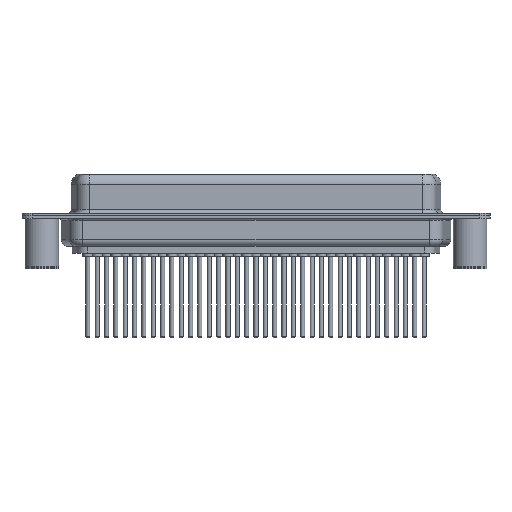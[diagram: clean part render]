
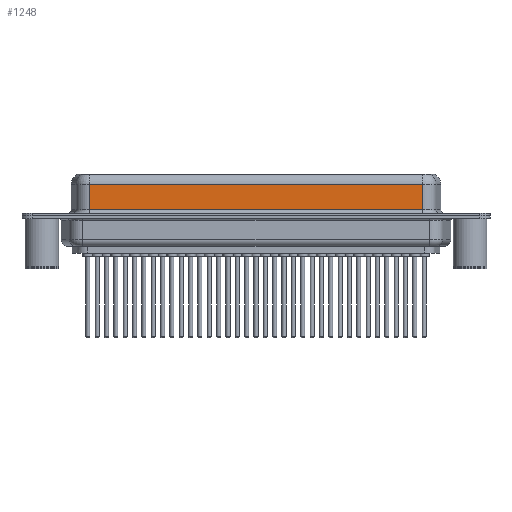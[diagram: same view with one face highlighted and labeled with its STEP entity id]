
A CAD part, front view. The second image highlights one B-rep face of the part: STEP entity #1248.
In plain terms, the highlighted planar face has unit normal (0, -1, 0).
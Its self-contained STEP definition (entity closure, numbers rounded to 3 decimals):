
#472 = CARTESIAN_POINT ( 'NONE',  ( 7.038, -3.95, 4.65 ) ) ;
#1124 = LINE ( 'NONE', #24276, #9348 ) ;
#1248 = ADVANCED_FACE ( 'NONE', ( #10222 ), #18622, .F. ) ;
#1699 = LINE ( 'NONE', #10457, #20418 ) ;
#3807 = EDGE_LOOP ( 'NONE', ( #18335, #27020, #5341, #15226 ) ) ;
#4194 = VERTEX_POINT ( 'NONE', #5720 ) ;
#5341 = ORIENTED_EDGE ( 'NONE', *, *, #24609, .T. ) ;
#5720 = CARTESIAN_POINT ( 'NONE',  ( 7.038, -3.95, 0.9 ) ) ;
#5757 = DIRECTION ( 'NONE',  ( 0., 0., -1. ) ) ;
#5765 = CARTESIAN_POINT ( 'NONE',  ( 56.462, -3.95, 6.4 ) ) ;
#7512 = VERTEX_POINT ( 'NONE', #19748 ) ;
#7856 = AXIS2_PLACEMENT_3D ( 'NONE', #26952, #8157, #16528 ) ;
#7986 = CARTESIAN_POINT ( 'NONE',  ( 56.462, -3.95, 0.9 ) ) ;
#8157 = DIRECTION ( 'NONE',  ( 0., 1., 0. ) ) ;
#9348 = VECTOR ( 'NONE', #9733, 1000. ) ;
#9733 = DIRECTION ( 'NONE',  ( 1., 0., 0. ) ) ;
#9814 = CARTESIAN_POINT ( 'NONE',  ( 7.038, -3.95, 6.4 ) ) ;
#10222 = FACE_OUTER_BOUND ( 'NONE', #3807, .T. ) ;
#10275 = VERTEX_POINT ( 'NONE', #472 ) ;
#10457 = CARTESIAN_POINT ( 'NONE',  ( 56.462, -3.95, 4.65 ) ) ;
#14700 = EDGE_CURVE ( 'NONE', #7512, #18676, #24625, .T. ) ;
#15202 = VECTOR ( 'NONE', #5757, 1000. ) ;
#15226 = ORIENTED_EDGE ( 'NONE', *, *, #16273, .T. ) ;
#16262 = LINE ( 'NONE', #9814, #15202 ) ;
#16273 = EDGE_CURVE ( 'NONE', #4194, #18676, #1124, .T. ) ;
#16528 = DIRECTION ( 'NONE',  ( -1., 0., 0. ) ) ;
#17682 = VECTOR ( 'NONE', #24922, 1000. ) ;
#18335 = ORIENTED_EDGE ( 'NONE', *, *, #14700, .F. ) ;
#18622 = PLANE ( 'NONE',  #7856 ) ;
#18676 = VERTEX_POINT ( 'NONE', #7986 ) ;
#18992 = DIRECTION ( 'NONE',  ( -1., 0., 0. ) ) ;
#19748 = CARTESIAN_POINT ( 'NONE',  ( 56.462, -3.95, 4.65 ) ) ;
#20418 = VECTOR ( 'NONE', #18992, 1000. ) ;
#20481 = EDGE_CURVE ( 'NONE', #7512, #10275, #1699, .T. ) ;
#24276 = CARTESIAN_POINT ( 'NONE',  ( 56.462, -3.95, 0.9 ) ) ;
#24609 = EDGE_CURVE ( 'NONE', #10275, #4194, #16262, .T. ) ;
#24625 = LINE ( 'NONE', #5765, #17682 ) ;
#24922 = DIRECTION ( 'NONE',  ( 0., 0., -1. ) ) ;
#26952 = CARTESIAN_POINT ( 'NONE',  ( 56.462, -3.95, 6.4 ) ) ;
#27020 = ORIENTED_EDGE ( 'NONE', *, *, #20481, .T. ) ;
